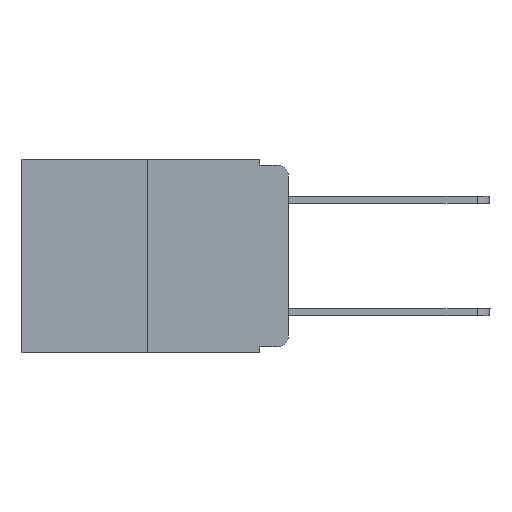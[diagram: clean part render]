
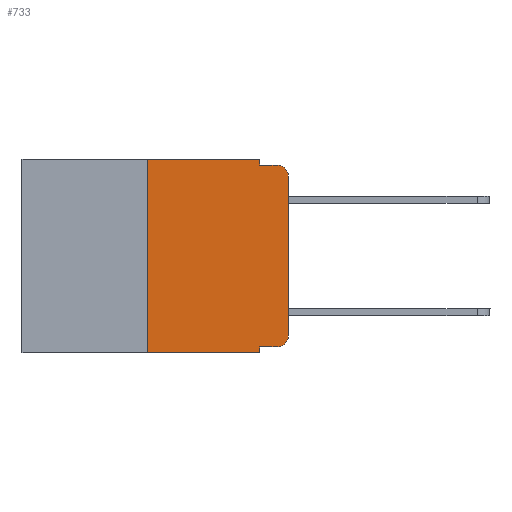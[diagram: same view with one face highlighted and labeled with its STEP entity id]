
A CAD part, left-side view. The second image highlights one B-rep face of the part: STEP entity #733.
In plain terms, the highlighted planar face has unit normal (-1, 0, 0).
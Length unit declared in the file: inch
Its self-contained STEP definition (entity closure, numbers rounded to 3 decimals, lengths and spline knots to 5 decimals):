
#558 = EDGE_CURVE ( 'NONE', #598, #657, #5115, .T. ) ;
#598 = VERTEX_POINT ( 'NONE', #3957 ) ;
#620 = ORIENTED_EDGE ( 'NONE', *, *, #558, .T. ) ;
#657 = VERTEX_POINT ( 'NONE', #2138 ) ;
#733 = ADVANCED_FACE ( 'NONE', ( #11648 ), #1718, .F. ) ;
#860 = DIRECTION ( 'NONE',  ( 0., 0., -1. ) ) ;
#986 = CARTESIAN_POINT ( 'NONE',  ( 0., 0.051, 0. ) ) ;
#1050 = DIRECTION ( 'NONE',  ( 0., 0., -1. ) ) ;
#1373 = LINE ( 'NONE', #7713, #10578 ) ;
#1419 = DIRECTION ( 'NONE',  ( 0., 0., 1. ) ) ;
#1718 = PLANE ( 'NONE',  #4337 ) ;
#1821 = CARTESIAN_POINT ( 'NONE',  ( 0., 0.02, -0.01 ) ) ;
#2089 = ORIENTED_EDGE ( 'NONE', *, *, #2302, .F. ) ;
#2138 = CARTESIAN_POINT ( 'NONE',  ( 0., 0.02, -0.333 ) ) ;
#2275 = CARTESIAN_POINT ( 'NONE',  ( 0., 0.25, -0.343 ) ) ;
#2301 = DIRECTION ( 'NONE',  ( 0., 0., 1. ) ) ;
#2302 = EDGE_CURVE ( 'NONE', #5895, #10777, #1373, .T. ) ;
#2383 = ORIENTED_EDGE ( 'NONE', *, *, #3357, .T. ) ;
#2394 = LINE ( 'NONE', #2981, #7322 ) ;
#2553 = EDGE_CURVE ( 'NONE', #7969, #10676, #6629, .T. ) ;
#2708 = ORIENTED_EDGE ( 'NONE', *, *, #2553, .F. ) ;
#2939 = DIRECTION ( 'NONE',  ( 1., 0., 0. ) ) ;
#2981 = CARTESIAN_POINT ( 'NONE',  ( 0., 0.473, 0. ) ) ;
#3025 = CARTESIAN_POINT ( 'NONE',  ( 0., 0., -0.313 ) ) ;
#3055 = CARTESIAN_POINT ( 'NONE',  ( 0., 0.051, -0.01 ) ) ;
#3078 = CARTESIAN_POINT ( 'NONE',  ( 0., 0.051, 0. ) ) ;
#3141 = EDGE_CURVE ( 'NONE', #10676, #5895, #2394, .T. ) ;
#3341 = EDGE_CURVE ( 'NONE', #598, #10205, #8356, .T. ) ;
#3357 = EDGE_CURVE ( 'NONE', #7969, #10205, #5901, .T. ) ;
#3442 = ORIENTED_EDGE ( 'NONE', *, *, #3341, .F. ) ;
#3862 = AXIS2_PLACEMENT_3D ( 'NONE', #6060, #9765, #5988 ) ;
#3957 = CARTESIAN_POINT ( 'NONE',  ( 0., 0.051, -0.333 ) ) ;
#4077 = DIRECTION ( 'NONE',  ( 0., -1., 0. ) ) ;
#4337 = AXIS2_PLACEMENT_3D ( 'NONE', #4698, #2939, #4881 ) ;
#4698 = CARTESIAN_POINT ( 'NONE',  ( 0., 0.473, 0. ) ) ;
#4777 = CARTESIAN_POINT ( 'NONE',  ( 0., 0.02, -0.03 ) ) ;
#4881 = DIRECTION ( 'NONE',  ( 0., 0., -1. ) ) ;
#5115 = LINE ( 'NONE', #6153, #11773 ) ;
#5185 = CIRCLE ( 'NONE', #9302, 0.02 ) ;
#5326 = ORIENTED_EDGE ( 'NONE', *, *, #9318, .T. ) ;
#5432 = ORIENTED_EDGE ( 'NONE', *, *, #3141, .F. ) ;
#5895 = VERTEX_POINT ( 'NONE', #3078 ) ;
#5901 = LINE ( 'NONE', #12028, #8927 ) ;
#5908 = VERTEX_POINT ( 'NONE', #6779 ) ;
#5988 = DIRECTION ( 'NONE',  ( 0., 0., -1. ) ) ;
#6060 = CARTESIAN_POINT ( 'NONE',  ( 0., 0.02, -0.313 ) ) ;
#6153 = CARTESIAN_POINT ( 'NONE',  ( 0., 0.051, -0.333 ) ) ;
#6444 = VERTEX_POINT ( 'NONE', #3025 ) ;
#6531 = EDGE_CURVE ( 'NONE', #10777, #7416, #11448, .T. ) ;
#6629 = LINE ( 'NONE', #6947, #7483 ) ;
#6653 = EDGE_CURVE ( 'NONE', #6444, #5908, #8382, .T. ) ;
#6779 = CARTESIAN_POINT ( 'NONE',  ( 0., 0., -0.03 ) ) ;
#6947 = CARTESIAN_POINT ( 'NONE',  ( 0., 0.25, 0. ) ) ;
#7020 = CARTESIAN_POINT ( 'NONE',  ( 0., 0., 0. ) ) ;
#7075 = DIRECTION ( 'NONE',  ( 0., -1., 0. ) ) ;
#7086 = VECTOR ( 'NONE', #1419, 39.37008 ) ;
#7322 = VECTOR ( 'NONE', #10547, 39.37008 ) ;
#7416 = VERTEX_POINT ( 'NONE', #1821 ) ;
#7483 = VECTOR ( 'NONE', #2301, 39.37008 ) ;
#7507 = ORIENTED_EDGE ( 'NONE', *, *, #6653, .T. ) ;
#7713 = CARTESIAN_POINT ( 'NONE',  ( 0., 0.051, 0. ) ) ;
#7942 = VECTOR ( 'NONE', #860, 39.37008 ) ;
#7969 = VERTEX_POINT ( 'NONE', #2275 ) ;
#8047 = ORIENTED_EDGE ( 'NONE', *, *, #6531, .F. ) ;
#8356 = LINE ( 'NONE', #986, #7942 ) ;
#8382 = LINE ( 'NONE', #7020, #7086 ) ;
#8383 = DIRECTION ( 'NONE',  ( 0., 0., -1. ) ) ;
#8604 = CARTESIAN_POINT ( 'NONE',  ( 0., 0.25, 0. ) ) ;
#8927 = VECTOR ( 'NONE', #10271, 39.37008 ) ;
#9248 = DIRECTION ( 'NONE',  ( -1., 0., 0. ) ) ;
#9302 = AXIS2_PLACEMENT_3D ( 'NONE', #4777, #9248, #8383 ) ;
#9318 = EDGE_CURVE ( 'NONE', #657, #6444, #10513, .T. ) ;
#9765 = DIRECTION ( 'NONE',  ( -1., 0., 0. ) ) ;
#10004 = ORIENTED_EDGE ( 'NONE', *, *, #11132, .T. ) ;
#10205 = VERTEX_POINT ( 'NONE', #11875 ) ;
#10271 = DIRECTION ( 'NONE',  ( 0., -1., 0. ) ) ;
#10513 = CIRCLE ( 'NONE', #3862, 0.02 ) ;
#10547 = DIRECTION ( 'NONE',  ( 0., -1., 0. ) ) ;
#10559 = EDGE_LOOP ( 'NONE', ( #7507, #10004, #8047, #2089, #5432, #2708, #2383, #3442, #620, #5326 ) ) ;
#10578 = VECTOR ( 'NONE', #1050, 39.37008 ) ;
#10661 = CARTESIAN_POINT ( 'NONE',  ( 0., 0.051, -0.01 ) ) ;
#10676 = VERTEX_POINT ( 'NONE', #8604 ) ;
#10777 = VERTEX_POINT ( 'NONE', #10661 ) ;
#11132 = EDGE_CURVE ( 'NONE', #5908, #7416, #5185, .T. ) ;
#11289 = VECTOR ( 'NONE', #4077, 39.37008 ) ;
#11448 = LINE ( 'NONE', #3055, #11289 ) ;
#11648 = FACE_OUTER_BOUND ( 'NONE', #10559, .T. ) ;
#11773 = VECTOR ( 'NONE', #7075, 39.37008 ) ;
#11875 = CARTESIAN_POINT ( 'NONE',  ( 0., 0.051, -0.343 ) ) ;
#12028 = CARTESIAN_POINT ( 'NONE',  ( 0., 0.473, -0.343 ) ) ;
